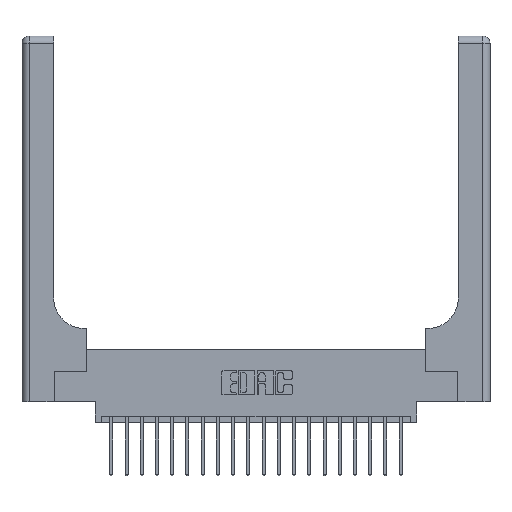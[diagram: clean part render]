
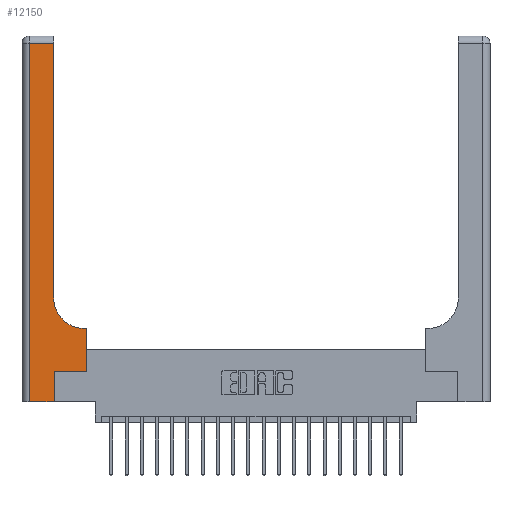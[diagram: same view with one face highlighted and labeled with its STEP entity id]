
A CAD part, top view. The second image highlights one B-rep face of the part: STEP entity #12150.
In plain terms, the highlighted planar face has unit normal (0, 0, 1).
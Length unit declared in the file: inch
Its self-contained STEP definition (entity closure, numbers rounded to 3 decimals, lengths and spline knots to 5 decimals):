
#188 = CARTESIAN_POINT ( 'NONE',  ( 0.26, 2.94, 0.37 ) ) ;
#381 = VECTOR ( 'NONE', #18749, 39.37008 ) ;
#905 = VERTEX_POINT ( 'NONE', #11732 ) ;
#1004 = VERTEX_POINT ( 'NONE', #5578 ) ;
#1212 = DIRECTION ( 'NONE',  ( 0., 0., -1. ) ) ;
#1323 = FACE_OUTER_BOUND ( 'NONE', #2139, .T. ) ;
#1544 = PLANE ( 'NONE',  #6697 ) ;
#1625 = EDGE_CURVE ( 'NONE', #12715, #10147, #2662, .T. ) ;
#1796 = LINE ( 'NONE', #11514, #9276 ) ;
#2139 = EDGE_LOOP ( 'NONE', ( #15763, #11401, #17132, #17392, #6614, #8118, #11540, #9455, #13891 ) ) ;
#2335 = LINE ( 'NONE', #19195, #381 ) ;
#2388 = DIRECTION ( 'NONE',  ( 0., 1., 0. ) ) ;
#2574 = DIRECTION ( 'NONE',  ( 1., 0., 0. ) ) ;
#2662 = LINE ( 'NONE', #4767, #3621 ) ;
#2857 = CARTESIAN_POINT ( 'NONE',  ( 0., 2.94, 0.37 ) ) ;
#3051 = AXIS2_PLACEMENT_3D ( 'NONE', #16536, #18075, #9709 ) ;
#3621 = VECTOR ( 'NONE', #14548, 39.37008 ) ;
#3648 = VERTEX_POINT ( 'NONE', #13423 ) ;
#3748 = EDGE_CURVE ( 'NONE', #19533, #15894, #14069, .T. ) ;
#3801 = CARTESIAN_POINT ( 'NONE',  ( 0.265, 0.25, 0.37 ) ) ;
#4212 = CARTESIAN_POINT ( 'NONE',  ( 0.26, 3., 0.37 ) ) ;
#4428 = VECTOR ( 'NONE', #2388, 39.37008 ) ;
#4649 = DIRECTION ( 'NONE',  ( -1., 0., 0. ) ) ;
#4732 = EDGE_CURVE ( 'NONE', #3648, #1004, #12551, .T. ) ;
#4767 = CARTESIAN_POINT ( 'NONE',  ( 0.06, 3., 0.37 ) ) ;
#5028 = DIRECTION ( 'NONE',  ( 1., 0., 0. ) ) ;
#5578 = CARTESIAN_POINT ( 'NONE',  ( 0.26, 0.85, 0.37 ) ) ;
#6614 = ORIENTED_EDGE ( 'NONE', *, *, #9499, .T. ) ;
#6697 = AXIS2_PLACEMENT_3D ( 'NONE', #9710, #1212, #4649 ) ;
#7397 = EDGE_CURVE ( 'NONE', #15894, #3648, #2335, .T. ) ;
#7963 = EDGE_CURVE ( 'NONE', #9609, #12715, #13105, .T. ) ;
#8118 = ORIENTED_EDGE ( 'NONE', *, *, #15960, .T. ) ;
#9276 = VECTOR ( 'NONE', #5028, 39.37008 ) ;
#9365 = LINE ( 'NONE', #12880, #19530 ) ;
#9455 = ORIENTED_EDGE ( 'NONE', *, *, #7397, .T. ) ;
#9499 = EDGE_CURVE ( 'NONE', #905, #12629, #9365, .T. ) ;
#9609 = VERTEX_POINT ( 'NONE', #188 ) ;
#9709 = DIRECTION ( 'NONE',  ( 1., 0., 0. ) ) ;
#9710 = CARTESIAN_POINT ( 'NONE',  ( 0., 3., 0.37 ) ) ;
#10147 = VERTEX_POINT ( 'NONE', #14000 ) ;
#10733 = LINE ( 'NONE', #21224, #13074 ) ;
#11401 = ORIENTED_EDGE ( 'NONE', *, *, #7963, .T. ) ;
#11514 = CARTESIAN_POINT ( 'NONE',  ( 0., 0., 0.37 ) ) ;
#11540 = ORIENTED_EDGE ( 'NONE', *, *, #3748, .T. ) ;
#11732 = CARTESIAN_POINT ( 'NONE',  ( 0.265, 0., 0.37 ) ) ;
#11951 = CARTESIAN_POINT ( 'NONE',  ( 0.528, 0.6, 0.37 ) ) ;
#12130 = EDGE_CURVE ( 'NONE', #1004, #9609, #19294, .T. ) ;
#12150 = ADVANCED_FACE ( 'NONE', ( #1323 ), #1544, .F. ) ;
#12551 = CIRCLE ( 'NONE', #3051, 0.25 ) ;
#12629 = VERTEX_POINT ( 'NONE', #3801 ) ;
#12715 = VERTEX_POINT ( 'NONE', #13814 ) ;
#12880 = CARTESIAN_POINT ( 'NONE',  ( 0.265, 0., 0.37 ) ) ;
#13074 = VECTOR ( 'NONE', #2574, 39.37008 ) ;
#13105 = LINE ( 'NONE', #2857, #13138 ) ;
#13138 = VECTOR ( 'NONE', #21183, 39.37008 ) ;
#13423 = CARTESIAN_POINT ( 'NONE',  ( 0.51, 0.6, 0.37 ) ) ;
#13814 = CARTESIAN_POINT ( 'NONE',  ( 0.06, 2.94, 0.37 ) ) ;
#13891 = ORIENTED_EDGE ( 'NONE', *, *, #4732, .T. ) ;
#14000 = CARTESIAN_POINT ( 'NONE',  ( 0.06, 0., 0.37 ) ) ;
#14069 = LINE ( 'NONE', #20699, #4428 ) ;
#14548 = DIRECTION ( 'NONE',  ( 0., -1., 0. ) ) ;
#14769 = DIRECTION ( 'NONE',  ( 0., 1., 0. ) ) ;
#15763 = ORIENTED_EDGE ( 'NONE', *, *, #12130, .T. ) ;
#15894 = VERTEX_POINT ( 'NONE', #11951 ) ;
#15960 = EDGE_CURVE ( 'NONE', #12629, #19533, #10733, .T. ) ;
#16536 = CARTESIAN_POINT ( 'NONE',  ( 0.51, 0.85, 0.37 ) ) ;
#16748 = CARTESIAN_POINT ( 'NONE',  ( 0.528, 0.25, 0.37 ) ) ;
#17132 = ORIENTED_EDGE ( 'NONE', *, *, #1625, .T. ) ;
#17260 = VECTOR ( 'NONE', #14769, 39.37008 ) ;
#17392 = ORIENTED_EDGE ( 'NONE', *, *, #20063, .T. ) ;
#18075 = DIRECTION ( 'NONE',  ( 0., 0., -1. ) ) ;
#18749 = DIRECTION ( 'NONE',  ( -1., 0., 0. ) ) ;
#19195 = CARTESIAN_POINT ( 'NONE',  ( 0.26, 0.6, 0.37 ) ) ;
#19294 = LINE ( 'NONE', #4212, #17260 ) ;
#19530 = VECTOR ( 'NONE', #21592, 39.37008 ) ;
#19533 = VERTEX_POINT ( 'NONE', #16748 ) ;
#20063 = EDGE_CURVE ( 'NONE', #10147, #905, #1796, .T. ) ;
#20699 = CARTESIAN_POINT ( 'NONE',  ( 0.528, 0.25, 0.37 ) ) ;
#21183 = DIRECTION ( 'NONE',  ( -1., 0., 0. ) ) ;
#21224 = CARTESIAN_POINT ( 'NONE',  ( 0.265, 0.25, 0.37 ) ) ;
#21592 = DIRECTION ( 'NONE',  ( 0., 1., 0. ) ) ;
